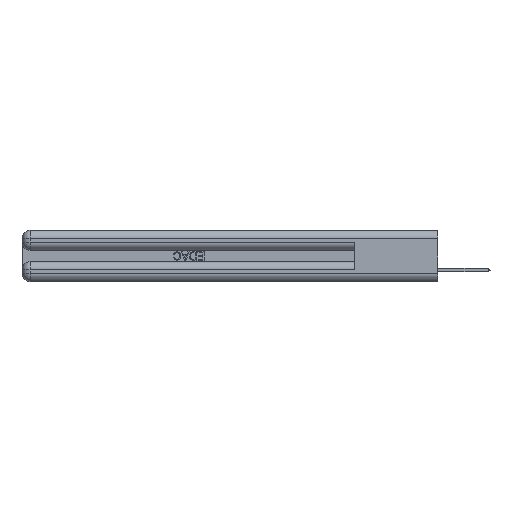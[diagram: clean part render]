
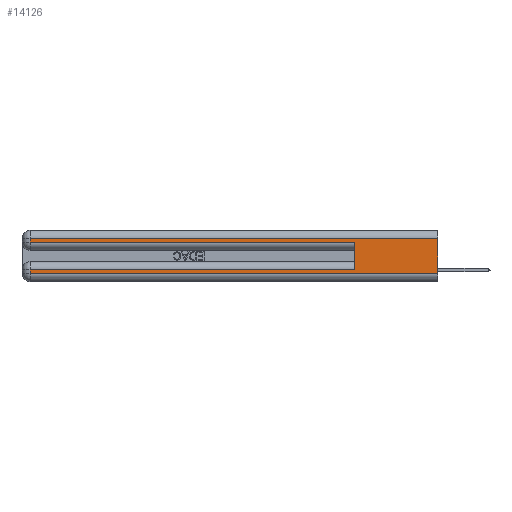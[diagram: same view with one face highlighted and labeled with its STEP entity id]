
A CAD part, left-side view. The second image highlights one B-rep face of the part: STEP entity #14126.
In plain terms, the highlighted planar face has unit normal (-1, 0, 0).
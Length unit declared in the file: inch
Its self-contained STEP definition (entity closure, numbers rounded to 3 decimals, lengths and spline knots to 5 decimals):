
#2524 = EDGE_CURVE ( 'NONE', #36043, #43694, #15682, .T. ) ;
#3357 = ORIENTED_EDGE ( 'NONE', *, *, #44561, .T. ) ;
#3369 = EDGE_CURVE ( 'NONE', #11354, #20811, #29098, .T. ) ;
#4207 = VERTEX_POINT ( 'NONE', #15469 ) ;
#5079 = VERTEX_POINT ( 'NONE', #38767 ) ;
#5697 = LINE ( 'NONE', #31031, #27643 ) ;
#7519 = LINE ( 'NONE', #25325, #36744 ) ;
#8326 = CARTESIAN_POINT ( 'NONE',  ( 0., 0., 0.085 ) ) ;
#8840 = LINE ( 'NONE', #23599, #35311 ) ;
#9201 = DIRECTION ( 'NONE',  ( 0., -1., 0. ) ) ;
#10406 = CARTESIAN_POINT ( 'NONE',  ( 0., 2.94, 0.085 ) ) ;
#10861 = VECTOR ( 'NONE', #44572, 39.37008 ) ;
#11354 = VERTEX_POINT ( 'NONE', #10406 ) ;
#12196 = EDGE_CURVE ( 'NONE', #27498, #11354, #39801, .T. ) ;
#13101 = DIRECTION ( 'NONE',  ( 1., 0., 0. ) ) ;
#13326 = EDGE_LOOP ( 'NONE', ( #38971, #32069, #39469, #3357, #30486, #34164, #27933, #37883 ) ) ;
#14126 = ADVANCED_FACE ( 'NONE', ( #45359 ), #35100, .F. ) ;
#15469 = CARTESIAN_POINT ( 'NONE',  ( 0., 2.94, 0.285 ) ) ;
#15682 = LINE ( 'NONE', #25937, #37641 ) ;
#16685 = CARTESIAN_POINT ( 'NONE',  ( 0., 2.94, 0.37 ) ) ;
#16833 = CARTESIAN_POINT ( 'NONE',  ( 0., 0., 0.37 ) ) ;
#17681 = DIRECTION ( 'NONE',  ( 0., 0., -1. ) ) ;
#19369 = CARTESIAN_POINT ( 'NONE',  ( 0., 0., 0.06 ) ) ;
#20252 = EDGE_CURVE ( 'NONE', #36043, #40844, #7519, .T. ) ;
#20657 = DIRECTION ( 'NONE',  ( 0., 0., -1. ) ) ;
#20811 = VERTEX_POINT ( 'NONE', #46656 ) ;
#21347 = DIRECTION ( 'NONE',  ( 0., 0., -1. ) ) ;
#21509 = CARTESIAN_POINT ( 'NONE',  ( 0., 2.94, 0.31 ) ) ;
#23599 = CARTESIAN_POINT ( 'NONE',  ( 0., 0., 0.285 ) ) ;
#23647 = LINE ( 'NONE', #19369, #29259 ) ;
#25325 = CARTESIAN_POINT ( 'NONE',  ( 0., 0., 0.37 ) ) ;
#25937 = CARTESIAN_POINT ( 'NONE',  ( 0., 0., 0.31 ) ) ;
#27498 = VERTEX_POINT ( 'NONE', #38322 ) ;
#27643 = VECTOR ( 'NONE', #20657, 39.37008 ) ;
#27933 = ORIENTED_EDGE ( 'NONE', *, *, #3369, .T. ) ;
#29098 = LINE ( 'NONE', #16685, #46013 ) ;
#29259 = VECTOR ( 'NONE', #9201, 39.37008 ) ;
#29262 = DIRECTION ( 'NONE',  ( 0., 1., 0. ) ) ;
#30173 = DIRECTION ( 'NONE',  ( 0., 1., 0. ) ) ;
#30486 = ORIENTED_EDGE ( 'NONE', *, *, #35403, .F. ) ;
#30714 = DIRECTION ( 'NONE',  ( 0., -1., 0. ) ) ;
#31031 = CARTESIAN_POINT ( 'NONE',  ( 0., 2.94, 0.37 ) ) ;
#31836 = EDGE_CURVE ( 'NONE', #43694, #4207, #5697, .T. ) ;
#31841 = CARTESIAN_POINT ( 'NONE',  ( 0., 0., 0.31 ) ) ;
#32069 = ORIENTED_EDGE ( 'NONE', *, *, #2524, .T. ) ;
#32130 = EDGE_CURVE ( 'NONE', #20811, #40844, #23647, .T. ) ;
#34164 = ORIENTED_EDGE ( 'NONE', *, *, #12196, .T. ) ;
#34235 = VECTOR ( 'NONE', #30173, 39.37008 ) ;
#35100 = PLANE ( 'NONE',  #35286 ) ;
#35286 = AXIS2_PLACEMENT_3D ( 'NONE', #16833, #13101, #42283 ) ;
#35311 = VECTOR ( 'NONE', #30714, 39.37008 ) ;
#35403 = EDGE_CURVE ( 'NONE', #27498, #5079, #41159, .T. ) ;
#36043 = VERTEX_POINT ( 'NONE', #31841 ) ;
#36744 = VECTOR ( 'NONE', #17681, 39.37008 ) ;
#37641 = VECTOR ( 'NONE', #29262, 39.37008 ) ;
#37883 = ORIENTED_EDGE ( 'NONE', *, *, #32130, .T. ) ;
#38322 = CARTESIAN_POINT ( 'NONE',  ( 0., 0.6, 0.085 ) ) ;
#38767 = CARTESIAN_POINT ( 'NONE',  ( 0., 0.6, 0.285 ) ) ;
#38971 = ORIENTED_EDGE ( 'NONE', *, *, #20252, .F. ) ;
#39469 = ORIENTED_EDGE ( 'NONE', *, *, #31836, .T. ) ;
#39801 = LINE ( 'NONE', #8326, #34235 ) ;
#40643 = CARTESIAN_POINT ( 'NONE',  ( 0., 0.6, 0.145 ) ) ;
#40844 = VERTEX_POINT ( 'NONE', #43764 ) ;
#41159 = LINE ( 'NONE', #40643, #10861 ) ;
#42283 = DIRECTION ( 'NONE',  ( 0., 0., -1. ) ) ;
#43694 = VERTEX_POINT ( 'NONE', #21509 ) ;
#43764 = CARTESIAN_POINT ( 'NONE',  ( 0., 0., 0.06 ) ) ;
#44561 = EDGE_CURVE ( 'NONE', #4207, #5079, #8840, .T. ) ;
#44572 = DIRECTION ( 'NONE',  ( 0., 0., 1. ) ) ;
#45359 = FACE_OUTER_BOUND ( 'NONE', #13326, .T. ) ;
#46013 = VECTOR ( 'NONE', #21347, 39.37008 ) ;
#46656 = CARTESIAN_POINT ( 'NONE',  ( 0., 2.94, 0.06 ) ) ;
